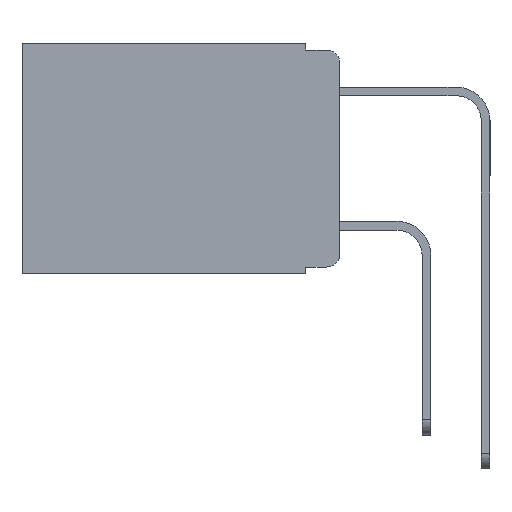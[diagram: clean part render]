
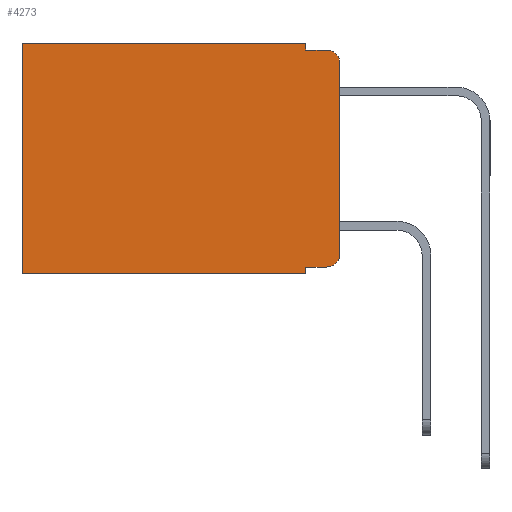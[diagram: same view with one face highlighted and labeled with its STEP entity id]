
A CAD part, left-side view. The second image highlights one B-rep face of the part: STEP entity #4273.
In plain terms, the highlighted planar face has unit normal (-1, 0, 0).
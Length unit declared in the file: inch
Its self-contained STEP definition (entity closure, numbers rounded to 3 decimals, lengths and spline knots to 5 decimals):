
#92 = CARTESIAN_POINT ( 'NONE',  ( 0.298, 0.051, -0.333 ) ) ;
#106 = CARTESIAN_POINT ( 'NONE',  ( 0.298, 0.051, -0.01 ) ) ;
#462 = VERTEX_POINT ( 'NONE', #1209 ) ;
#512 = CARTESIAN_POINT ( 'NONE',  ( 0.298, 0., 0. ) ) ;
#758 = VECTOR ( 'NONE', #12933, 39.37008 ) ;
#824 = CIRCLE ( 'NONE', #2734, 0.02 ) ;
#1044 = EDGE_CURVE ( 'NONE', #11871, #14315, #9435, .T. ) ;
#1209 = CARTESIAN_POINT ( 'NONE',  ( 0.298, 0., -0.03 ) ) ;
#1455 = AXIS2_PLACEMENT_3D ( 'NONE', #12236, #23993, #21314 ) ;
#1572 = EDGE_CURVE ( 'NONE', #18851, #4118, #7373, .T. ) ;
#2078 = ORIENTED_EDGE ( 'NONE', *, *, #12146, .F. ) ;
#2432 = VERTEX_POINT ( 'NONE', #11191 ) ;
#2734 = AXIS2_PLACEMENT_3D ( 'NONE', #9449, #22409, #11322 ) ;
#3422 = EDGE_CURVE ( 'NONE', #462, #11846, #19833, .T. ) ;
#3677 = LINE ( 'NONE', #10786, #21824 ) ;
#3850 = CARTESIAN_POINT ( 'NONE',  ( 0.298, 0.473, 0. ) ) ;
#3985 = CARTESIAN_POINT ( 'NONE',  ( 0.298, 0.02, -0.333 ) ) ;
#4118 = VERTEX_POINT ( 'NONE', #3985 ) ;
#4273 = ADVANCED_FACE ( 'NONE', ( #5511 ), #11851, .F. ) ;
#5463 = LINE ( 'NONE', #17632, #24094 ) ;
#5511 = FACE_OUTER_BOUND ( 'NONE', #9590, .T. ) ;
#5898 = LINE ( 'NONE', #20292, #758 ) ;
#6240 = EDGE_CURVE ( 'NONE', #18851, #2432, #21489, .T. ) ;
#6344 = DIRECTION ( 'NONE',  ( 0., 0., -1. ) ) ;
#6649 = DIRECTION ( 'NONE',  ( 0., -1., 0. ) ) ;
#6662 = DIRECTION ( 'NONE',  ( 0., 0., -1. ) ) ;
#7029 = VERTEX_POINT ( 'NONE', #106 ) ;
#7373 = LINE ( 'NONE', #22964, #16076 ) ;
#7527 = ORIENTED_EDGE ( 'NONE', *, *, #1572, .T. ) ;
#8093 = ORIENTED_EDGE ( 'NONE', *, *, #9120, .T. ) ;
#8695 = CARTESIAN_POINT ( 'NONE',  ( 0.298, 0.473, 0. ) ) ;
#8891 = CARTESIAN_POINT ( 'NONE',  ( 0.298, 0., 0. ) ) ;
#9120 = EDGE_CURVE ( 'NONE', #14315, #14246, #14076, .T. ) ;
#9390 = CARTESIAN_POINT ( 'NONE',  ( 0.298, 0.473, -0.343 ) ) ;
#9435 = LINE ( 'NONE', #21530, #23058 ) ;
#9449 = CARTESIAN_POINT ( 'NONE',  ( 0.298, 0.02, -0.313 ) ) ;
#9505 = DIRECTION ( 'NONE',  ( 0., 1., 0. ) ) ;
#9590 = EDGE_LOOP ( 'NONE', ( #15608, #9862, #21423, #18225, #15034, #8093, #2078, #19987, #7527, #16535 ) ) ;
#9778 = VECTOR ( 'NONE', #23520, 39.37008 ) ;
#9862 = ORIENTED_EDGE ( 'NONE', *, *, #3422, .T. ) ;
#9893 = CARTESIAN_POINT ( 'NONE',  ( 0.298, 0.02, -0.01 ) ) ;
#10292 = AXIS2_PLACEMENT_3D ( 'NONE', #512, #17501, #6344 ) ;
#10786 = CARTESIAN_POINT ( 'NONE',  ( 0.298, 0., -0.343 ) ) ;
#11191 = CARTESIAN_POINT ( 'NONE',  ( 0.298, 0.051, -0.343 ) ) ;
#11322 = DIRECTION ( 'NONE',  ( 0., 0., -1. ) ) ;
#11846 = VERTEX_POINT ( 'NONE', #9893 ) ;
#11851 = PLANE ( 'NONE',  #10292 ) ;
#11871 = VERTEX_POINT ( 'NONE', #21104 ) ;
#12146 = EDGE_CURVE ( 'NONE', #2432, #14246, #3677, .T. ) ;
#12211 = CARTESIAN_POINT ( 'NONE',  ( 0.298, 0., -0.313 ) ) ;
#12236 = CARTESIAN_POINT ( 'NONE',  ( 0.298, 0.02, -0.03 ) ) ;
#12933 = DIRECTION ( 'NONE',  ( 0., 0., -1. ) ) ;
#14076 = LINE ( 'NONE', #8695, #9778 ) ;
#14246 = VERTEX_POINT ( 'NONE', #9390 ) ;
#14315 = VERTEX_POINT ( 'NONE', #3850 ) ;
#15034 = ORIENTED_EDGE ( 'NONE', *, *, #1044, .T. ) ;
#15608 = ORIENTED_EDGE ( 'NONE', *, *, #21809, .F. ) ;
#16076 = VECTOR ( 'NONE', #17958, 39.37008 ) ;
#16535 = ORIENTED_EDGE ( 'NONE', *, *, #20553, .T. ) ;
#17129 = VECTOR ( 'NONE', #6662, 39.37008 ) ;
#17501 = DIRECTION ( 'NONE',  ( 1., 0., 0. ) ) ;
#17632 = CARTESIAN_POINT ( 'NONE',  ( 0.298, 0.051, -0.01 ) ) ;
#17811 = CARTESIAN_POINT ( 'NONE',  ( 0.298, 0.051, 0. ) ) ;
#17958 = DIRECTION ( 'NONE',  ( 0., -1., 0. ) ) ;
#18076 = VERTEX_POINT ( 'NONE', #12211 ) ;
#18141 = LINE ( 'NONE', #8891, #22513 ) ;
#18176 = DIRECTION ( 'NONE',  ( 0., 1., 0. ) ) ;
#18225 = ORIENTED_EDGE ( 'NONE', *, *, #21923, .F. ) ;
#18851 = VERTEX_POINT ( 'NONE', #92 ) ;
#19833 = CIRCLE ( 'NONE', #1455, 0.02 ) ;
#19987 = ORIENTED_EDGE ( 'NONE', *, *, #6240, .F. ) ;
#20292 = CARTESIAN_POINT ( 'NONE',  ( 0.298, 0.051, 0. ) ) ;
#20553 = EDGE_CURVE ( 'NONE', #4118, #18076, #824, .T. ) ;
#21104 = CARTESIAN_POINT ( 'NONE',  ( 0.298, 0.051, 0. ) ) ;
#21314 = DIRECTION ( 'NONE',  ( 0., 0., -1. ) ) ;
#21423 = ORIENTED_EDGE ( 'NONE', *, *, #23914, .F. ) ;
#21489 = LINE ( 'NONE', #17811, #17129 ) ;
#21530 = CARTESIAN_POINT ( 'NONE',  ( 0.298, 0., 0. ) ) ;
#21809 = EDGE_CURVE ( 'NONE', #462, #18076, #18141, .T. ) ;
#21824 = VECTOR ( 'NONE', #18176, 39.37008 ) ;
#21923 = EDGE_CURVE ( 'NONE', #11871, #7029, #5898, .T. ) ;
#22409 = DIRECTION ( 'NONE',  ( -1., 0., 0. ) ) ;
#22513 = VECTOR ( 'NONE', #23715, 39.37008 ) ;
#22964 = CARTESIAN_POINT ( 'NONE',  ( 0.298, 0.051, -0.333 ) ) ;
#23058 = VECTOR ( 'NONE', #9505, 39.37008 ) ;
#23520 = DIRECTION ( 'NONE',  ( 0., 0., -1. ) ) ;
#23715 = DIRECTION ( 'NONE',  ( 0., 0., -1. ) ) ;
#23914 = EDGE_CURVE ( 'NONE', #7029, #11846, #5463, .T. ) ;
#23993 = DIRECTION ( 'NONE',  ( -1., 0., 0. ) ) ;
#24094 = VECTOR ( 'NONE', #6649, 39.37008 ) ;
